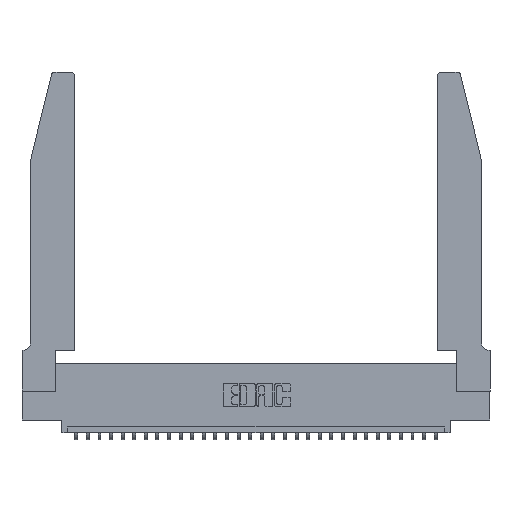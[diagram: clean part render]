
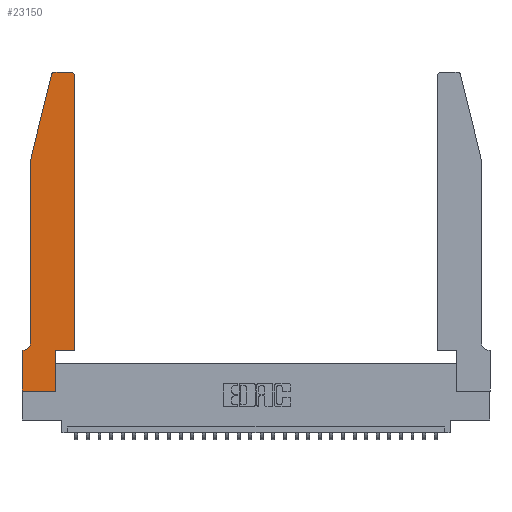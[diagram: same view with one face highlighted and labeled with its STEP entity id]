
A CAD part, top view. The second image highlights one B-rep face of the part: STEP entity #23150.
In plain terms, the highlighted planar face has unit normal (0, 0, 1).
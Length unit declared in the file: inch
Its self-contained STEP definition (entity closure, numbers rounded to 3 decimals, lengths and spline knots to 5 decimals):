
#82 = DIRECTION ( 'NONE',  ( 0., 1., 0. ) ) ;
#154 = AXIS2_PLACEMENT_3D ( 'NONE', #11520, #23631, #27963 ) ;
#242 = ORIENTED_EDGE ( 'NONE', *, *, #21079, .T. ) ;
#392 = CARTESIAN_POINT ( 'NONE',  ( 0.4505, 0.35, 0.37 ) ) ;
#986 = DIRECTION ( 'NONE',  ( 1., 0., 0. ) ) ;
#1692 = LINE ( 'NONE', #8983, #6815 ) ;
#2017 = AXIS2_PLACEMENT_3D ( 'NONE', #7230, #11818, #27839 ) ;
#2389 = CIRCLE ( 'NONE', #154, 0.03 ) ;
#2461 = CARTESIAN_POINT ( 'NONE',  ( 0.4505, 0.35, 0.37 ) ) ;
#2524 = CARTESIAN_POINT ( 'NONE',  ( 0.4205, 2.75, 0.37 ) ) ;
#3151 = EDGE_CURVE ( 'NONE', #24074, #9642, #1692, .T. ) ;
#3278 = VERTEX_POINT ( 'NONE', #16334 ) ;
#3282 = ORIENTED_EDGE ( 'NONE', *, *, #24313, .T. ) ;
#3515 = VERTEX_POINT ( 'NONE', #10728 ) ;
#4184 = VERTEX_POINT ( 'NONE', #20520 ) ;
#4257 = CARTESIAN_POINT ( 'NONE',  ( 0., 0., 0.37 ) ) ;
#4344 = EDGE_CURVE ( 'NONE', #10223, #12503, #18446, .T. ) ;
#4455 = CARTESIAN_POINT ( 'NONE',  ( 0.4505, 2.72, 0.37 ) ) ;
#4521 = ORIENTED_EDGE ( 'NONE', *, *, #4344, .T. ) ;
#5035 = ORIENTED_EDGE ( 'NONE', *, *, #14088, .T. ) ;
#5209 = AXIS2_PLACEMENT_3D ( 'NONE', #24297, #14785, #986 ) ;
#5288 = VECTOR ( 'NONE', #16770, 39.37008 ) ;
#5370 = EDGE_CURVE ( 'NONE', #3278, #4184, #24245, .T. ) ;
#5901 = DIRECTION ( 'NONE',  ( 1., 0., 0. ) ) ;
#6081 = VERTEX_POINT ( 'NONE', #30078 ) ;
#6645 = ORIENTED_EDGE ( 'NONE', *, *, #5370, .T. ) ;
#6815 = VECTOR ( 'NONE', #25603, 39.37008 ) ;
#7230 = CARTESIAN_POINT ( 'NONE',  ( 0.4205, 2.72, 0.37 ) ) ;
#8007 = PLANE ( 'NONE',  #5209 ) ;
#8322 = DIRECTION ( 'NONE',  ( -1., 0., 0. ) ) ;
#8351 = VECTOR ( 'NONE', #82, 39.37008 ) ;
#8949 = LINE ( 'NONE', #24443, #29538 ) ;
#8983 = CARTESIAN_POINT ( 'NONE',  ( 0.0755, 0.35, 0.37 ) ) ;
#9007 = VERTEX_POINT ( 'NONE', #28094 ) ;
#9642 = VERTEX_POINT ( 'NONE', #25920 ) ;
#9828 = LINE ( 'NONE', #2461, #8351 ) ;
#10223 = VERTEX_POINT ( 'NONE', #4455 ) ;
#10718 = CARTESIAN_POINT ( 'NONE',  ( 0.0055, 0.35, 0.37 ) ) ;
#10728 = CARTESIAN_POINT ( 'NONE',  ( 0.284, 2.75, 0.37 ) ) ;
#11021 = VECTOR ( 'NONE', #18157, 39.37008 ) ;
#11192 = LINE ( 'NONE', #16129, #29195 ) ;
#11317 = DIRECTION ( 'NONE',  ( -0.239, -0.971, 0. ) ) ;
#11520 = CARTESIAN_POINT ( 'NONE',  ( 0.284, 2.72, 0.37 ) ) ;
#11818 = DIRECTION ( 'NONE',  ( 0., 0., 1. ) ) ;
#11963 = EDGE_CURVE ( 'NONE', #12503, #3515, #13184, .T. ) ;
#12503 = VERTEX_POINT ( 'NONE', #2524 ) ;
#12522 = VECTOR ( 'NONE', #11317, 39.37008 ) ;
#13020 = CARTESIAN_POINT ( 'NONE',  ( 0.2865, 0.35, 0.37 ) ) ;
#13184 = LINE ( 'NONE', #24413, #20145 ) ;
#13472 = CARTESIAN_POINT ( 'NONE',  ( 0.0755, 2., 0.37 ) ) ;
#13764 = DIRECTION ( 'NONE',  ( 0., 1., 0. ) ) ;
#14088 = EDGE_CURVE ( 'NONE', #3515, #3278, #2389, .T. ) ;
#14340 = LINE ( 'NONE', #4257, #19102 ) ;
#14785 = DIRECTION ( 'NONE',  ( 0., 0., 1. ) ) ;
#15738 = CARTESIAN_POINT ( 'NONE',  ( 0.0755, 2., 0.37 ) ) ;
#16129 = CARTESIAN_POINT ( 'NONE',  ( 0.2865, 0.35, 0.37 ) ) ;
#16334 = CARTESIAN_POINT ( 'NONE',  ( 0.25487, 2.72718, 0.37 ) ) ;
#16519 = FACE_OUTER_BOUND ( 'NONE', #19547, .T. ) ;
#16770 = DIRECTION ( 'NONE',  ( 1., 0., 0. ) ) ;
#17016 = ORIENTED_EDGE ( 'NONE', *, *, #18838, .T. ) ;
#18048 = VERTEX_POINT ( 'NONE', #18622 ) ;
#18157 = DIRECTION ( 'NONE',  ( 0., -1., 0. ) ) ;
#18330 = EDGE_CURVE ( 'NONE', #30346, #24074, #28102, .T. ) ;
#18446 = CIRCLE ( 'NONE', #2017, 0.03 ) ;
#18622 = CARTESIAN_POINT ( 'NONE',  ( 0.4505, 0.35, 0.37 ) ) ;
#18838 = EDGE_CURVE ( 'NONE', #6081, #27184, #11192, .T. ) ;
#19102 = VECTOR ( 'NONE', #25346, 39.37008 ) ;
#19547 = EDGE_LOOP ( 'NONE', ( #21486, #5035, #6645, #21600, #28129, #24892, #22240, #27309, #17016, #242, #3282, #4521 ) ) ;
#20145 = VECTOR ( 'NONE', #24615, 39.37008 ) ;
#20520 = CARTESIAN_POINT ( 'NONE',  ( 0.0755, 2., 0.37 ) ) ;
#21079 = EDGE_CURVE ( 'NONE', #27184, #18048, #25085, .T. ) ;
#21486 = ORIENTED_EDGE ( 'NONE', *, *, #11963, .T. ) ;
#21600 = ORIENTED_EDGE ( 'NONE', *, *, #22766, .T. ) ;
#22240 = ORIENTED_EDGE ( 'NONE', *, *, #22874, .T. ) ;
#22550 = CARTESIAN_POINT ( 'NONE',  ( 0.0055, 0.42, 0.37 ) ) ;
#22766 = EDGE_CURVE ( 'NONE', #4184, #30346, #27560, .T. ) ;
#22874 = EDGE_CURVE ( 'NONE', #9642, #9007, #14340, .T. ) ;
#23150 = ADVANCED_FACE ( 'NONE', ( #16519 ), #8007, .T. ) ;
#23535 = AXIS2_PLACEMENT_3D ( 'NONE', #22550, #27407, #8322 ) ;
#23631 = DIRECTION ( 'NONE',  ( 0., 0., 1. ) ) ;
#24074 = VERTEX_POINT ( 'NONE', #10718 ) ;
#24245 = LINE ( 'NONE', #15738, #12522 ) ;
#24297 = CARTESIAN_POINT ( 'NONE',  ( 0., 0.35, 0.37 ) ) ;
#24313 = EDGE_CURVE ( 'NONE', #18048, #10223, #9828, .T. ) ;
#24413 = CARTESIAN_POINT ( 'NONE',  ( 0.2605, 2.75, 0.37 ) ) ;
#24443 = CARTESIAN_POINT ( 'NONE',  ( 0., 0., 0.37 ) ) ;
#24615 = DIRECTION ( 'NONE',  ( -1., 0., 0. ) ) ;
#24892 = ORIENTED_EDGE ( 'NONE', *, *, #3151, .T. ) ;
#25085 = LINE ( 'NONE', #392, #5288 ) ;
#25346 = DIRECTION ( 'NONE',  ( 0., -1., 0. ) ) ;
#25603 = DIRECTION ( 'NONE',  ( -1., 0., 0. ) ) ;
#25920 = CARTESIAN_POINT ( 'NONE',  ( 0., 0.35, 0.37 ) ) ;
#26067 = EDGE_CURVE ( 'NONE', #9007, #6081, #8949, .T. ) ;
#27184 = VERTEX_POINT ( 'NONE', #13020 ) ;
#27309 = ORIENTED_EDGE ( 'NONE', *, *, #26067, .T. ) ;
#27407 = DIRECTION ( 'NONE',  ( 0., 0., -1. ) ) ;
#27560 = LINE ( 'NONE', #13472, #11021 ) ;
#27839 = DIRECTION ( 'NONE',  ( 1., 0., 0. ) ) ;
#27963 = DIRECTION ( 'NONE',  ( 1., 0., 0. ) ) ;
#28094 = CARTESIAN_POINT ( 'NONE',  ( 0., 0., 0.37 ) ) ;
#28102 = CIRCLE ( 'NONE', #23535, 0.07 ) ;
#28129 = ORIENTED_EDGE ( 'NONE', *, *, #18330, .T. ) ;
#28475 = CARTESIAN_POINT ( 'NONE',  ( 0.0755, 0.42, 0.37 ) ) ;
#29195 = VECTOR ( 'NONE', #13764, 39.37008 ) ;
#29538 = VECTOR ( 'NONE', #5901, 39.37008 ) ;
#30078 = CARTESIAN_POINT ( 'NONE',  ( 0.2865, 0., 0.37 ) ) ;
#30346 = VERTEX_POINT ( 'NONE', #28475 ) ;
